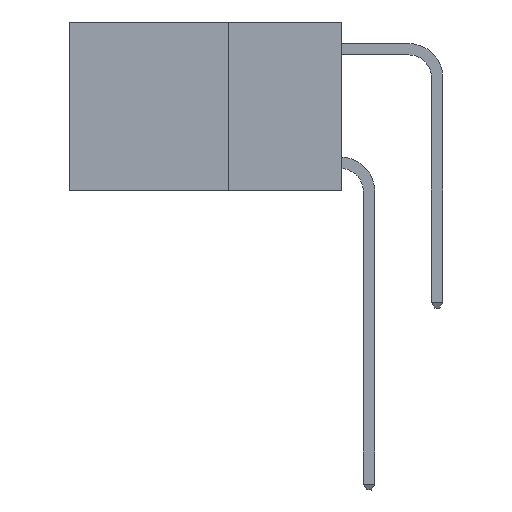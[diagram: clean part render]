
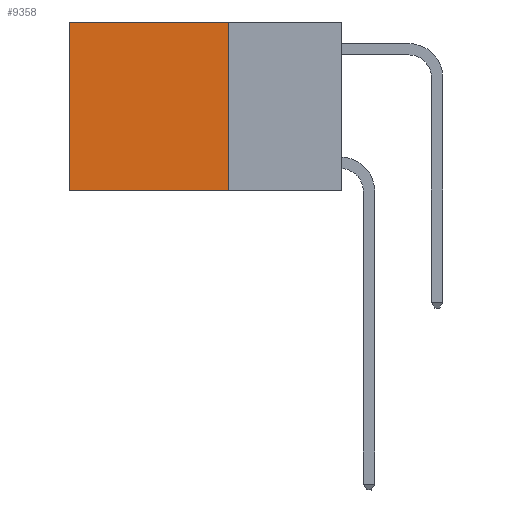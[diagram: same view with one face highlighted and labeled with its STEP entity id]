
A CAD part, left-side view. The second image highlights one B-rep face of the part: STEP entity #9358.
In plain terms, the highlighted planar face has unit normal (-1, 0, 0).
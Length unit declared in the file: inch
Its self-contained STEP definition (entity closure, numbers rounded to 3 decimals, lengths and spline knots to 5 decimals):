
#195 = VERTEX_POINT ( 'NONE', #13975 ) ;
#245 = ORIENTED_EDGE ( 'NONE', *, *, #19194, .T. ) ;
#1261 = EDGE_LOOP ( 'NONE', ( #245, #1590, #7719, #1670 ) ) ;
#1308 = CARTESIAN_POINT ( 'NONE',  ( 0.2625, 0.25, 0. ) ) ;
#1487 = EDGE_CURVE ( 'NONE', #195, #16485, #4072, .T. ) ;
#1590 = ORIENTED_EDGE ( 'NONE', *, *, #7226, .F. ) ;
#1670 = ORIENTED_EDGE ( 'NONE', *, *, #1487, .T. ) ;
#2645 = DIRECTION ( 'NONE',  ( 0., 0., -1. ) ) ;
#3341 = DIRECTION ( 'NONE',  ( 0., 0., -1. ) ) ;
#3436 = VECTOR ( 'NONE', #3987, 39.37008 ) ;
#3987 = DIRECTION ( 'NONE',  ( 0., 1., 0. ) ) ;
#4072 = LINE ( 'NONE', #17552, #3436 ) ;
#4274 = EDGE_CURVE ( 'NONE', #195, #24433, #11997, .T. ) ;
#5648 = CARTESIAN_POINT ( 'NONE',  ( 0.2625, 0.25, -0.37 ) ) ;
#6158 = CARTESIAN_POINT ( 'NONE',  ( 0.2625, 0.6, 0. ) ) ;
#6415 = LINE ( 'NONE', #6625, #16693 ) ;
#6625 = CARTESIAN_POINT ( 'NONE',  ( 0.2625, 0.6, 0. ) ) ;
#6831 = VECTOR ( 'NONE', #20746, 39.37008 ) ;
#7226 = EDGE_CURVE ( 'NONE', #24433, #17392, #25122, .T. ) ;
#7243 = PLANE ( 'NONE',  #16888 ) ;
#7719 = ORIENTED_EDGE ( 'NONE', *, *, #4274, .F. ) ;
#9358 = ADVANCED_FACE ( 'NONE', ( #18386 ), #7243, .F. ) ;
#11997 = LINE ( 'NONE', #24517, #6831 ) ;
#13975 = CARTESIAN_POINT ( 'NONE',  ( 0.2625, 0.25, 0. ) ) ;
#14346 = VECTOR ( 'NONE', #21118, 39.37008 ) ;
#15053 = DIRECTION ( 'NONE',  ( 1., 0., 0. ) ) ;
#16485 = VERTEX_POINT ( 'NONE', #6158 ) ;
#16693 = VECTOR ( 'NONE', #2645, 39.37008 ) ;
#16729 = CARTESIAN_POINT ( 'NONE',  ( 0.2625, 0.25, -0.37 ) ) ;
#16888 = AXIS2_PLACEMENT_3D ( 'NONE', #1308, #15053, #3341 ) ;
#17001 = CARTESIAN_POINT ( 'NONE',  ( 0.2625, 0.6, -0.37 ) ) ;
#17392 = VERTEX_POINT ( 'NONE', #17001 ) ;
#17552 = CARTESIAN_POINT ( 'NONE',  ( 0.2625, 0.25, 0. ) ) ;
#18386 = FACE_OUTER_BOUND ( 'NONE', #1261, .T. ) ;
#19194 = EDGE_CURVE ( 'NONE', #16485, #17392, #6415, .T. ) ;
#20746 = DIRECTION ( 'NONE',  ( 0., 0., -1. ) ) ;
#21118 = DIRECTION ( 'NONE',  ( 0., 1., 0. ) ) ;
#24433 = VERTEX_POINT ( 'NONE', #16729 ) ;
#24517 = CARTESIAN_POINT ( 'NONE',  ( 0.2625, 0.25, 0. ) ) ;
#25122 = LINE ( 'NONE', #5648, #14346 ) ;
